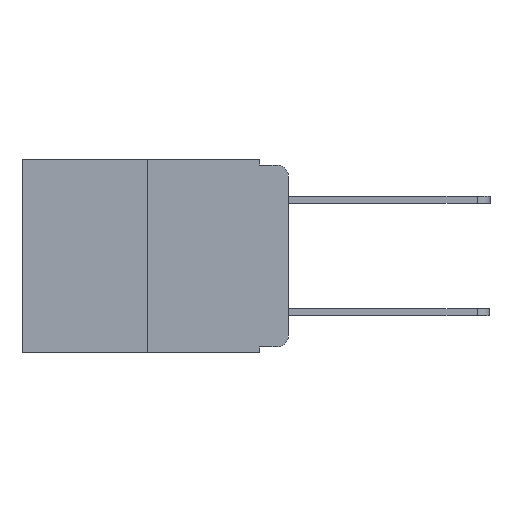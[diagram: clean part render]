
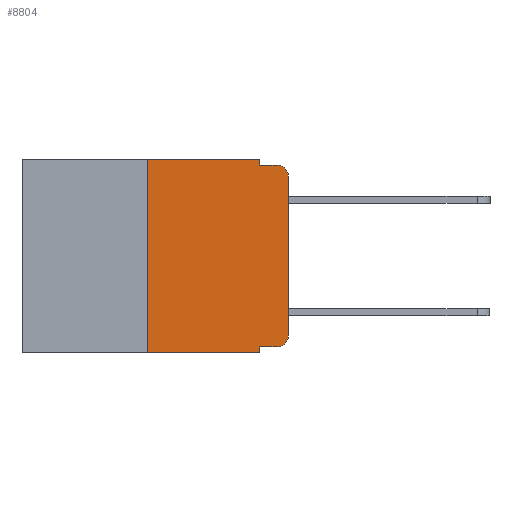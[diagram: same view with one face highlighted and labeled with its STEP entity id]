
A CAD part, left-side view. The second image highlights one B-rep face of the part: STEP entity #8804.
In plain terms, the highlighted planar face has unit normal (-1, 0, 0).
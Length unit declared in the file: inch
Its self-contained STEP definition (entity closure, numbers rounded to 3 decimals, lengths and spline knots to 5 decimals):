
#290 = CARTESIAN_POINT ( 'NONE',  ( 0., 0., -0.03 ) ) ;
#911 = LINE ( 'NONE', #6526, #9752 ) ;
#1435 = LINE ( 'NONE', #7919, #17848 ) ;
#1534 = VERTEX_POINT ( 'NONE', #8327 ) ;
#1586 = EDGE_CURVE ( 'NONE', #5944, #7177, #17155, .T. ) ;
#1758 = CARTESIAN_POINT ( 'NONE',  ( 0., 0.051, 0. ) ) ;
#2160 = EDGE_CURVE ( 'NONE', #5944, #12851, #14008, .T. ) ;
#2348 = CARTESIAN_POINT ( 'NONE',  ( 0., 0.051, -0.01 ) ) ;
#2498 = CARTESIAN_POINT ( 'NONE',  ( 0., 0.473, -0.343 ) ) ;
#2526 = VERTEX_POINT ( 'NONE', #6489 ) ;
#2532 = CARTESIAN_POINT ( 'NONE',  ( 0., 0.25, 0. ) ) ;
#2731 = EDGE_CURVE ( 'NONE', #5690, #1534, #4442, .T. ) ;
#3041 = ORIENTED_EDGE ( 'NONE', *, *, #16751, .F. ) ;
#3401 = DIRECTION ( 'NONE',  ( 0., 0., -1. ) ) ;
#3463 = CARTESIAN_POINT ( 'NONE',  ( 0., 0.051, -0.333 ) ) ;
#3657 = CARTESIAN_POINT ( 'NONE',  ( 0., 0.02, -0.03 ) ) ;
#4294 = AXIS2_PLACEMENT_3D ( 'NONE', #3657, #14855, #5301 ) ;
#4295 = ORIENTED_EDGE ( 'NONE', *, *, #2731, .T. ) ;
#4442 = CIRCLE ( 'NONE', #4294, 0.02 ) ;
#4489 = VECTOR ( 'NONE', #14123, 39.37008 ) ;
#4816 = ORIENTED_EDGE ( 'NONE', *, *, #9881, .T. ) ;
#4955 = VECTOR ( 'NONE', #13135, 39.37008 ) ;
#5079 = FACE_OUTER_BOUND ( 'NONE', #18830, .T. ) ;
#5301 = DIRECTION ( 'NONE',  ( 0., 0., -1. ) ) ;
#5491 = LINE ( 'NONE', #1758, #9383 ) ;
#5690 = VERTEX_POINT ( 'NONE', #290 ) ;
#5944 = VERTEX_POINT ( 'NONE', #12380 ) ;
#5977 = DIRECTION ( 'NONE',  ( -1., 0., 0. ) ) ;
#6400 = ORIENTED_EDGE ( 'NONE', *, *, #6703, .F. ) ;
#6489 = CARTESIAN_POINT ( 'NONE',  ( 0., 0.051, -0.333 ) ) ;
#6526 = CARTESIAN_POINT ( 'NONE',  ( 0., 0.473, 0. ) ) ;
#6703 = EDGE_CURVE ( 'NONE', #10304, #12026, #13180, .T. ) ;
#7121 = VERTEX_POINT ( 'NONE', #16652 ) ;
#7164 = ORIENTED_EDGE ( 'NONE', *, *, #19309, .T. ) ;
#7177 = VERTEX_POINT ( 'NONE', #2532 ) ;
#7919 = CARTESIAN_POINT ( 'NONE',  ( 0., 0.051, -0.01 ) ) ;
#8327 = CARTESIAN_POINT ( 'NONE',  ( 0., 0.02, -0.01 ) ) ;
#8777 = CARTESIAN_POINT ( 'NONE',  ( 0., 0.051, 0. ) ) ;
#8804 = ADVANCED_FACE ( 'NONE', ( #5079 ), #17592, .F. ) ;
#8922 = LINE ( 'NONE', #17189, #4489 ) ;
#8977 = VERTEX_POINT ( 'NONE', #14949 ) ;
#9383 = VECTOR ( 'NONE', #3401, 39.37008 ) ;
#9752 = VECTOR ( 'NONE', #15986, 39.37008 ) ;
#9881 = EDGE_CURVE ( 'NONE', #7121, #8977, #16256, .T. ) ;
#9976 = DIRECTION ( 'NONE',  ( 1., 0., 0. ) ) ;
#10022 = EDGE_CURVE ( 'NONE', #12026, #1534, #1435, .T. ) ;
#10182 = DIRECTION ( 'NONE',  ( 0., 0., 1. ) ) ;
#10304 = VERTEX_POINT ( 'NONE', #8777 ) ;
#10599 = CARTESIAN_POINT ( 'NONE',  ( 0., 0.25, 0. ) ) ;
#11241 = AXIS2_PLACEMENT_3D ( 'NONE', #16109, #9976, #19904 ) ;
#12026 = VERTEX_POINT ( 'NONE', #2348 ) ;
#12380 = CARTESIAN_POINT ( 'NONE',  ( 0., 0.25, -0.343 ) ) ;
#12584 = VECTOR ( 'NONE', #10182, 39.37008 ) ;
#12640 = ORIENTED_EDGE ( 'NONE', *, *, #1586, .F. ) ;
#12851 = VERTEX_POINT ( 'NONE', #14960 ) ;
#13125 = ORIENTED_EDGE ( 'NONE', *, *, #2160, .T. ) ;
#13135 = DIRECTION ( 'NONE',  ( 0., -1., 0. ) ) ;
#13180 = LINE ( 'NONE', #18453, #13674 ) ;
#13611 = ORIENTED_EDGE ( 'NONE', *, *, #19255, .F. ) ;
#13674 = VECTOR ( 'NONE', #13993, 39.37008 ) ;
#13850 = ORIENTED_EDGE ( 'NONE', *, *, #10022, .F. ) ;
#13993 = DIRECTION ( 'NONE',  ( 0., 0., -1. ) ) ;
#14008 = LINE ( 'NONE', #2498, #17120 ) ;
#14123 = DIRECTION ( 'NONE',  ( 0., 0., 1. ) ) ;
#14855 = DIRECTION ( 'NONE',  ( -1., 0., 0. ) ) ;
#14949 = CARTESIAN_POINT ( 'NONE',  ( 0., 0., -0.313 ) ) ;
#14960 = CARTESIAN_POINT ( 'NONE',  ( 0., 0.051, -0.343 ) ) ;
#15439 = CARTESIAN_POINT ( 'NONE',  ( 0., 0.02, -0.313 ) ) ;
#15986 = DIRECTION ( 'NONE',  ( 0., -1., 0. ) ) ;
#16109 = CARTESIAN_POINT ( 'NONE',  ( 0., 0.473, 0. ) ) ;
#16256 = CIRCLE ( 'NONE', #19180, 0.02 ) ;
#16652 = CARTESIAN_POINT ( 'NONE',  ( 0., 0.02, -0.333 ) ) ;
#16751 = EDGE_CURVE ( 'NONE', #7177, #10304, #911, .T. ) ;
#16997 = DIRECTION ( 'NONE',  ( 0., 0., -1. ) ) ;
#17108 = LINE ( 'NONE', #3463, #4955 ) ;
#17120 = VECTOR ( 'NONE', #19670, 39.37008 ) ;
#17155 = LINE ( 'NONE', #10599, #12584 ) ;
#17189 = CARTESIAN_POINT ( 'NONE',  ( 0., 0., 0. ) ) ;
#17240 = DIRECTION ( 'NONE',  ( 0., -1., 0. ) ) ;
#17592 = PLANE ( 'NONE',  #11241 ) ;
#17848 = VECTOR ( 'NONE', #17240, 39.37008 ) ;
#18405 = EDGE_CURVE ( 'NONE', #8977, #5690, #8922, .T. ) ;
#18453 = CARTESIAN_POINT ( 'NONE',  ( 0., 0.051, 0. ) ) ;
#18830 = EDGE_LOOP ( 'NONE', ( #19895, #4295, #13850, #6400, #3041, #12640, #13125, #13611, #7164, #4816 ) ) ;
#19180 = AXIS2_PLACEMENT_3D ( 'NONE', #15439, #5977, #16997 ) ;
#19255 = EDGE_CURVE ( 'NONE', #2526, #12851, #5491, .T. ) ;
#19309 = EDGE_CURVE ( 'NONE', #2526, #7121, #17108, .T. ) ;
#19670 = DIRECTION ( 'NONE',  ( 0., -1., 0. ) ) ;
#19895 = ORIENTED_EDGE ( 'NONE', *, *, #18405, .T. ) ;
#19904 = DIRECTION ( 'NONE',  ( 0., 0., -1. ) ) ;
